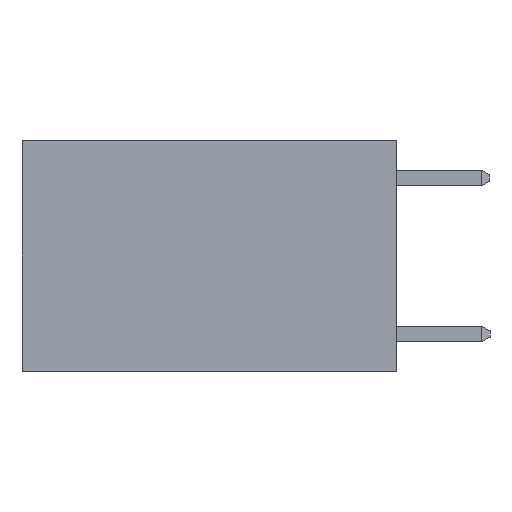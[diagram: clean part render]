
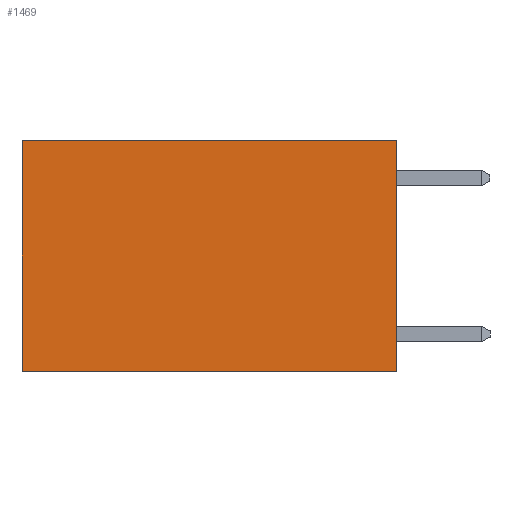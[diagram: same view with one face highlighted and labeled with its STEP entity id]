
A CAD part, left-side view. The second image highlights one B-rep face of the part: STEP entity #1469.
In plain terms, the highlighted planar face has unit normal (-1, 0, 0).
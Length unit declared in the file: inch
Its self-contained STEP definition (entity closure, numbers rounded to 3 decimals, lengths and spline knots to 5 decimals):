
#290 = LINE ( 'NONE', #4441, #6966 ) ;
#380 = EDGE_CURVE ( 'NONE', #1498, #1166, #290, .T. ) ;
#845 = ORIENTED_EDGE ( 'NONE', *, *, #6561, .F. ) ;
#1006 = LINE ( 'NONE', #8245, #5919 ) ;
#1166 = VERTEX_POINT ( 'NONE', #7588 ) ;
#1260 = ORIENTED_EDGE ( 'NONE', *, *, #7750, .T. ) ;
#1462 = CARTESIAN_POINT ( 'NONE',  ( 0.2625, 0.6, 0. ) ) ;
#1469 = ADVANCED_FACE ( 'NONE', ( #2765 ), #5346, .F. ) ;
#1498 = VERTEX_POINT ( 'NONE', #4101 ) ;
#2550 = DIRECTION ( 'NONE',  ( 0., 0., -1. ) ) ;
#2765 = FACE_OUTER_BOUND ( 'NONE', #3121, .T. ) ;
#2824 = DIRECTION ( 'NONE',  ( 0., 0., -1. ) ) ;
#3121 = EDGE_LOOP ( 'NONE', ( #1260, #845, #6287, #8272 ) ) ;
#3281 = VERTEX_POINT ( 'NONE', #3458 ) ;
#3456 = CARTESIAN_POINT ( 'NONE',  ( 0.2625, 0., 0. ) ) ;
#3458 = CARTESIAN_POINT ( 'NONE',  ( 0.2625, 0.6, -0.37 ) ) ;
#3731 = DIRECTION ( 'NONE',  ( 0., 0., -1. ) ) ;
#4101 = CARTESIAN_POINT ( 'NONE',  ( 0.2625, 0., 0. ) ) ;
#4441 = CARTESIAN_POINT ( 'NONE',  ( 0.2625, 0., 0. ) ) ;
#4767 = DIRECTION ( 'NONE',  ( 0., 1., 0. ) ) ;
#5115 = CARTESIAN_POINT ( 'NONE',  ( 0.2625, 0., -0.37 ) ) ;
#5142 = LINE ( 'NONE', #5115, #8333 ) ;
#5317 = EDGE_CURVE ( 'NONE', #1498, #7371, #7957, .T. ) ;
#5346 = PLANE ( 'NONE',  #6373 ) ;
#5919 = VECTOR ( 'NONE', #2550, 39.37008 ) ;
#6274 = VECTOR ( 'NONE', #4767, 39.37008 ) ;
#6287 = ORIENTED_EDGE ( 'NONE', *, *, #380, .F. ) ;
#6373 = AXIS2_PLACEMENT_3D ( 'NONE', #3456, #6637, #2824 ) ;
#6561 = EDGE_CURVE ( 'NONE', #1166, #3281, #5142, .T. ) ;
#6637 = DIRECTION ( 'NONE',  ( 1., 0., 0. ) ) ;
#6966 = VECTOR ( 'NONE', #3731, 39.37008 ) ;
#7315 = CARTESIAN_POINT ( 'NONE',  ( 0.2625, 0., 0. ) ) ;
#7371 = VERTEX_POINT ( 'NONE', #1462 ) ;
#7588 = CARTESIAN_POINT ( 'NONE',  ( 0.2625, 0., -0.37 ) ) ;
#7750 = EDGE_CURVE ( 'NONE', #7371, #3281, #1006, .T. ) ;
#7957 = LINE ( 'NONE', #7315, #6274 ) ;
#8245 = CARTESIAN_POINT ( 'NONE',  ( 0.2625, 0.6, 0. ) ) ;
#8272 = ORIENTED_EDGE ( 'NONE', *, *, #5317, .T. ) ;
#8291 = DIRECTION ( 'NONE',  ( 0., 1., 0. ) ) ;
#8333 = VECTOR ( 'NONE', #8291, 39.37008 ) ;
